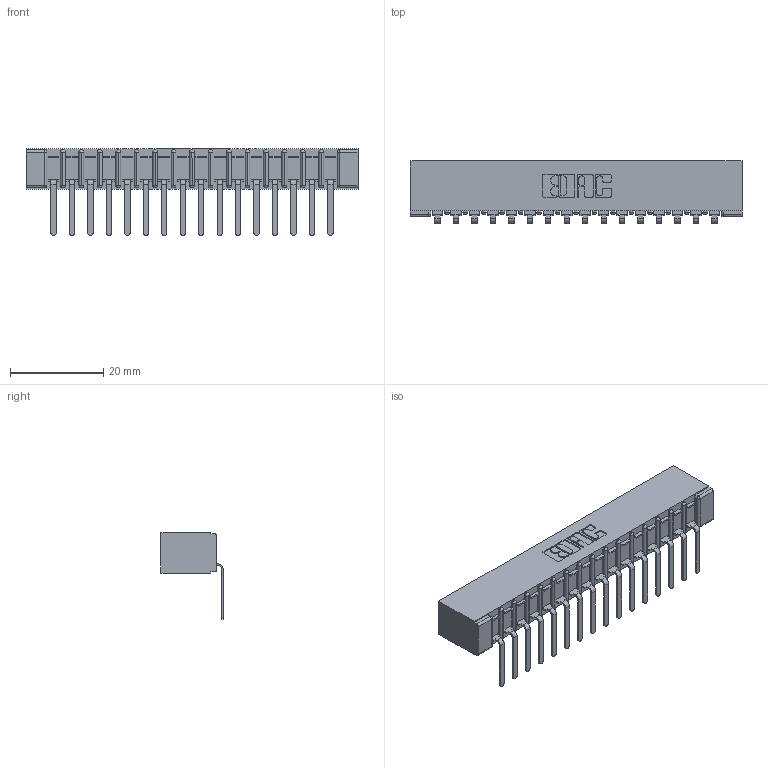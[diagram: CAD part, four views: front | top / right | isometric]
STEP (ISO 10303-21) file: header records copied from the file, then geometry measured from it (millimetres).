
FILE_DESCRIPTION (( 'STEP AP203' ), '1' );
FILE_NAME ('307-016-557-101.STEP', '2018-08-03T03:33:39', ( '' ), ( '' ), 'SwSTEP 2.0', 'SolidWorks 2016', '' );
FILE_SCHEMA (( 'CONFIG_CONTROL_DESIGN' ));
Length unit declared in the file: inch
Products named in the file (3): 307-016-557-101; 307 Part_No Mounting Lugs; 307-290-002_557
Assembly tree (17 placements, depth 2):
  307-016-557-101
    307 Part_No Mounting Lugs
    307-290-002_557  x16
Bounding box: 71.27 x 13.32 x 18.67 mm (x, y, z)
Volume: 4987.6 mm3; surface area: 9509.1 mm2
Topology: 17 solids, 17 shells, 1375 faces, 4203 edges, 2754 vertices
Faces by surface type: plane 818, cylinder 523, sphere 34
Entity records: 17498 total; most frequent: CARTESIAN_POINT 2948, ORIENTED_EDGE 2938, DIRECTION 2875, EDGE_CURVE 1469, LINE 1113, VECTOR 1113, VERTEX_POINT 954, AXIS2_PLACEMENT_3D 881
